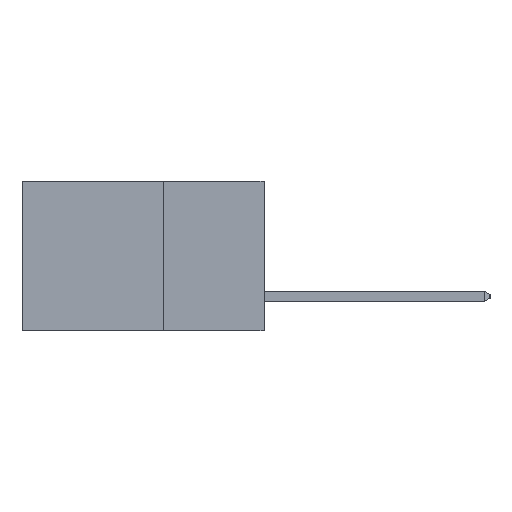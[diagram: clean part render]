
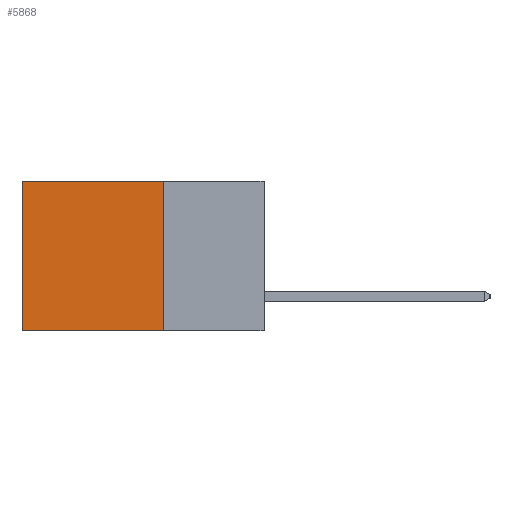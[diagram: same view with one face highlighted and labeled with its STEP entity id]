
A CAD part, left-side view. The second image highlights one B-rep face of the part: STEP entity #5868.
In plain terms, the highlighted planar face has unit normal (-1, 0, 0).
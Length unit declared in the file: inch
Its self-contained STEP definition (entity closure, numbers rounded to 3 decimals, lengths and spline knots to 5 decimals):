
#179 = CARTESIAN_POINT ( 'NONE',  ( 0.2615, 0.6, 0. ) ) ;
#345 = CARTESIAN_POINT ( 'NONE',  ( 0.2615, 0.25, -0.37 ) ) ;
#377 = LINE ( 'NONE', #7254, #8225 ) ;
#545 = VERTEX_POINT ( 'NONE', #179 ) ;
#603 = LINE ( 'NONE', #345, #4605 ) ;
#835 = VERTEX_POINT ( 'NONE', #7018 ) ;
#1117 = EDGE_CURVE ( 'NONE', #835, #3001, #2246, .T. ) ;
#1609 = ORIENTED_EDGE ( 'NONE', *, *, #3650, .T. ) ;
#1636 = ORIENTED_EDGE ( 'NONE', *, *, #6272, .F. ) ;
#1659 = ORIENTED_EDGE ( 'NONE', *, *, #1117, .F. ) ;
#1680 = ORIENTED_EDGE ( 'NONE', *, *, #3406, .T. ) ;
#2246 = LINE ( 'NONE', #9164, #7942 ) ;
#2425 = VECTOR ( 'NONE', #6253, 39.37008 ) ;
#3001 = VERTEX_POINT ( 'NONE', #9300 ) ;
#3167 = DIRECTION ( 'NONE',  ( 0., 0., -1. ) ) ;
#3197 = DIRECTION ( 'NONE',  ( 0., 0., -1. ) ) ;
#3265 = PLANE ( 'NONE',  #5400 ) ;
#3406 = EDGE_CURVE ( 'NONE', #835, #545, #377, .T. ) ;
#3650 = EDGE_CURVE ( 'NONE', #545, #4139, #8806, .T. ) ;
#3989 = CARTESIAN_POINT ( 'NONE',  ( 0.2615, 0.6, -0.37 ) ) ;
#4139 = VERTEX_POINT ( 'NONE', #3989 ) ;
#4306 = CARTESIAN_POINT ( 'NONE',  ( 0.2615, 0.25, -0.37 ) ) ;
#4562 = DIRECTION ( 'NONE',  ( 1., 0., 0. ) ) ;
#4605 = VECTOR ( 'NONE', #8948, 39.37008 ) ;
#5223 = EDGE_LOOP ( 'NONE', ( #1609, #1636, #1659, #1680 ) ) ;
#5400 = AXIS2_PLACEMENT_3D ( 'NONE', #4306, #4562, #3167 ) ;
#5868 = ADVANCED_FACE ( 'NONE', ( #9107 ), #3265, .F. ) ;
#6253 = DIRECTION ( 'NONE',  ( 0., 0., -1. ) ) ;
#6262 = CARTESIAN_POINT ( 'NONE',  ( 0.2615, 0.6, -0.37 ) ) ;
#6272 = EDGE_CURVE ( 'NONE', #3001, #4139, #603, .T. ) ;
#7018 = CARTESIAN_POINT ( 'NONE',  ( 0.2615, 0.25, 0. ) ) ;
#7251 = DIRECTION ( 'NONE',  ( 0., 1., 0. ) ) ;
#7254 = CARTESIAN_POINT ( 'NONE',  ( 0.2615, 0.25, 0. ) ) ;
#7942 = VECTOR ( 'NONE', #3197, 39.37008 ) ;
#8225 = VECTOR ( 'NONE', #7251, 39.37008 ) ;
#8806 = LINE ( 'NONE', #6262, #2425 ) ;
#8948 = DIRECTION ( 'NONE',  ( 0., 1., 0. ) ) ;
#9107 = FACE_OUTER_BOUND ( 'NONE', #5223, .T. ) ;
#9164 = CARTESIAN_POINT ( 'NONE',  ( 0.2615, 0.25, -0.37 ) ) ;
#9300 = CARTESIAN_POINT ( 'NONE',  ( 0.2615, 0.25, -0.37 ) ) ;
